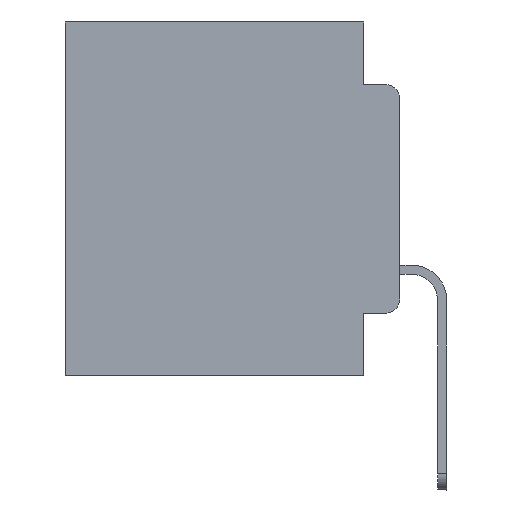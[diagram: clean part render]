
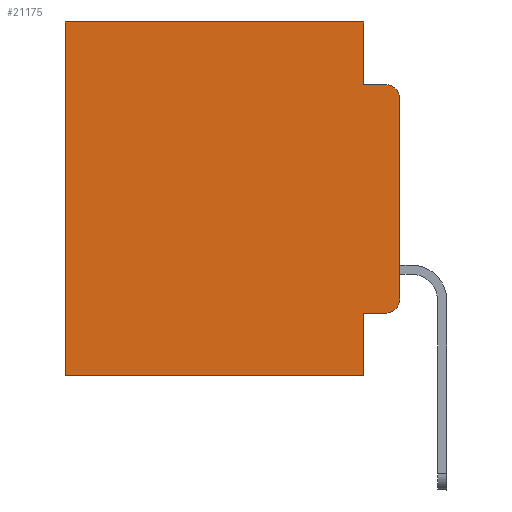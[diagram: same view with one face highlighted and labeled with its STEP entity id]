
A CAD part, left-side view. The second image highlights one B-rep face of the part: STEP entity #21175.
In plain terms, the highlighted planar face has unit normal (-1, 0, 0).
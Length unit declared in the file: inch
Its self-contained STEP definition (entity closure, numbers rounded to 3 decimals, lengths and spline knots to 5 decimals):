
#634 = ORIENTED_EDGE ( 'NONE', *, *, #6458, .T. ) ;
#723 = CARTESIAN_POINT ( 'NONE',  ( 0.298, 0., 0. ) ) ;
#1043 = VECTOR ( 'NONE', #14343, 39.37008 ) ;
#1610 = VECTOR ( 'NONE', #3441, 39.37008 ) ;
#1612 = ORIENTED_EDGE ( 'NONE', *, *, #3949, .F. ) ;
#1692 = ORIENTED_EDGE ( 'NONE', *, *, #13865, .T. ) ;
#1721 = ORIENTED_EDGE ( 'NONE', *, *, #2396, .F. ) ;
#2145 = CARTESIAN_POINT ( 'NONE',  ( 0.298, 0.051, -0.5 ) ) ;
#2396 = EDGE_CURVE ( 'NONE', #9184, #18791, #24381, .T. ) ;
#2931 = AXIS2_PLACEMENT_3D ( 'NONE', #22878, #9513, #15501 ) ;
#3113 = VERTEX_POINT ( 'NONE', #8367 ) ;
#3311 = VERTEX_POINT ( 'NONE', #8899 ) ;
#3441 = DIRECTION ( 'NONE',  ( 0., 1., 0. ) ) ;
#3834 = DIRECTION ( 'NONE',  ( 0., 0., -1. ) ) ;
#3949 = EDGE_CURVE ( 'NONE', #18791, #3311, #19730, .T. ) ;
#5088 = CARTESIAN_POINT ( 'NONE',  ( 0.298, 0.02, -0.4115 ) ) ;
#5637 = CARTESIAN_POINT ( 'NONE',  ( 0.298, 0., -0.5 ) ) ;
#5680 = CARTESIAN_POINT ( 'NONE',  ( 0.298, 0.051, -0.4115 ) ) ;
#6050 = LINE ( 'NONE', #19377, #22060 ) ;
#6451 = LINE ( 'NONE', #24295, #1043 ) ;
#6458 = EDGE_CURVE ( 'NONE', #23062, #3311, #7569, .T. ) ;
#7018 = DIRECTION ( 'NONE',  ( 0., 0., -1. ) ) ;
#7162 = AXIS2_PLACEMENT_3D ( 'NONE', #22114, #10299, #18208 ) ;
#7569 = LINE ( 'NONE', #23385, #23602 ) ;
#8367 = CARTESIAN_POINT ( 'NONE',  ( 0.298, 0.051, 0. ) ) ;
#8590 = CARTESIAN_POINT ( 'NONE',  ( 0.298, 0.051, 0. ) ) ;
#8899 = CARTESIAN_POINT ( 'NONE',  ( 0.298, 0.473, -0.5 ) ) ;
#8959 = CARTESIAN_POINT ( 'NONE',  ( 0.298, 0., 0. ) ) ;
#9109 = CIRCLE ( 'NONE', #2931, 0.02 ) ;
#9184 = VERTEX_POINT ( 'NONE', #5680 ) ;
#9484 = CARTESIAN_POINT ( 'NONE',  ( 0.298, 0.02, -0.0885 ) ) ;
#9513 = DIRECTION ( 'NONE',  ( -1., 0., 0. ) ) ;
#9550 = VERTEX_POINT ( 'NONE', #13657 ) ;
#9631 = EDGE_CURVE ( 'NONE', #10975, #11256, #13796, .T. ) ;
#9883 = DIRECTION ( 'NONE',  ( 0., -1., 0. ) ) ;
#10299 = DIRECTION ( 'NONE',  ( -1., 0., 0. ) ) ;
#10975 = VERTEX_POINT ( 'NONE', #12485 ) ;
#10985 = EDGE_CURVE ( 'NONE', #9184, #25526, #14313, .T. ) ;
#11256 = VERTEX_POINT ( 'NONE', #9484 ) ;
#11300 = CIRCLE ( 'NONE', #7162, 0.02 ) ;
#12345 = LINE ( 'NONE', #8959, #24440 ) ;
#12361 = CARTESIAN_POINT ( 'NONE',  ( 0.298, 0.051, -0.4115 ) ) ;
#12485 = CARTESIAN_POINT ( 'NONE',  ( 0.298, 0.051, -0.0885 ) ) ;
#12919 = VECTOR ( 'NONE', #7018, 39.37008 ) ;
#13212 = ORIENTED_EDGE ( 'NONE', *, *, #20829, .T. ) ;
#13657 = CARTESIAN_POINT ( 'NONE',  ( 0.298, 0., -0.1085 ) ) ;
#13796 = LINE ( 'NONE', #21704, #18690 ) ;
#13865 = EDGE_CURVE ( 'NONE', #3113, #23062, #12345, .T. ) ;
#13948 = DIRECTION ( 'NONE',  ( 0., 0., -1. ) ) ;
#14169 = PLANE ( 'NONE',  #18360 ) ;
#14313 = LINE ( 'NONE', #12361, #20033 ) ;
#14343 = DIRECTION ( 'NONE',  ( 0., 0., -1. ) ) ;
#14404 = CARTESIAN_POINT ( 'NONE',  ( 0.298, 0.473, 0. ) ) ;
#14913 = ORIENTED_EDGE ( 'NONE', *, *, #16226, .F. ) ;
#15501 = DIRECTION ( 'NONE',  ( 0., 0., -1. ) ) ;
#16226 = EDGE_CURVE ( 'NONE', #3113, #10975, #6050, .T. ) ;
#17122 = ORIENTED_EDGE ( 'NONE', *, *, #23551, .T. ) ;
#18208 = DIRECTION ( 'NONE',  ( 0., 0., -1. ) ) ;
#18306 = FACE_OUTER_BOUND ( 'NONE', #21024, .T. ) ;
#18360 = AXIS2_PLACEMENT_3D ( 'NONE', #723, #18447, #24262 ) ;
#18426 = CARTESIAN_POINT ( 'NONE',  ( 0.298, 0., -0.3915 ) ) ;
#18447 = DIRECTION ( 'NONE',  ( 1., 0., 0. ) ) ;
#18690 = VECTOR ( 'NONE', #9883, 39.37008 ) ;
#18791 = VERTEX_POINT ( 'NONE', #2145 ) ;
#19354 = ORIENTED_EDGE ( 'NONE', *, *, #9631, .F. ) ;
#19377 = CARTESIAN_POINT ( 'NONE',  ( 0.298, 0.051, 0. ) ) ;
#19730 = LINE ( 'NONE', #5637, #1610 ) ;
#20033 = VECTOR ( 'NONE', #20255, 39.37008 ) ;
#20255 = DIRECTION ( 'NONE',  ( 0., -1., 0. ) ) ;
#20829 = EDGE_CURVE ( 'NONE', #9550, #11256, #11300, .T. ) ;
#21024 = EDGE_LOOP ( 'NONE', ( #22154, #13212, #19354, #14913, #1692, #634, #1612, #1721, #21462, #17122 ) ) ;
#21175 = ADVANCED_FACE ( 'NONE', ( #18306 ), #14169, .F. ) ;
#21462 = ORIENTED_EDGE ( 'NONE', *, *, #10985, .T. ) ;
#21704 = CARTESIAN_POINT ( 'NONE',  ( 0.298, 0.051, -0.0885 ) ) ;
#22060 = VECTOR ( 'NONE', #13948, 39.37008 ) ;
#22086 = EDGE_CURVE ( 'NONE', #9550, #23006, #6451, .T. ) ;
#22114 = CARTESIAN_POINT ( 'NONE',  ( 0.298, 0.02, -0.1085 ) ) ;
#22154 = ORIENTED_EDGE ( 'NONE', *, *, #22086, .F. ) ;
#22878 = CARTESIAN_POINT ( 'NONE',  ( 0.298, 0.02, -0.3915 ) ) ;
#23006 = VERTEX_POINT ( 'NONE', #18426 ) ;
#23062 = VERTEX_POINT ( 'NONE', #14404 ) ;
#23385 = CARTESIAN_POINT ( 'NONE',  ( 0.298, 0.473, 0. ) ) ;
#23551 = EDGE_CURVE ( 'NONE', #25526, #23006, #9109, .T. ) ;
#23602 = VECTOR ( 'NONE', #3834, 39.37008 ) ;
#24262 = DIRECTION ( 'NONE',  ( 0., 0., -1. ) ) ;
#24295 = CARTESIAN_POINT ( 'NONE',  ( 0.298, 0., 0. ) ) ;
#24381 = LINE ( 'NONE', #8590, #12919 ) ;
#24440 = VECTOR ( 'NONE', #24492, 39.37008 ) ;
#24492 = DIRECTION ( 'NONE',  ( 0., 1., 0. ) ) ;
#25526 = VERTEX_POINT ( 'NONE', #5088 ) ;
